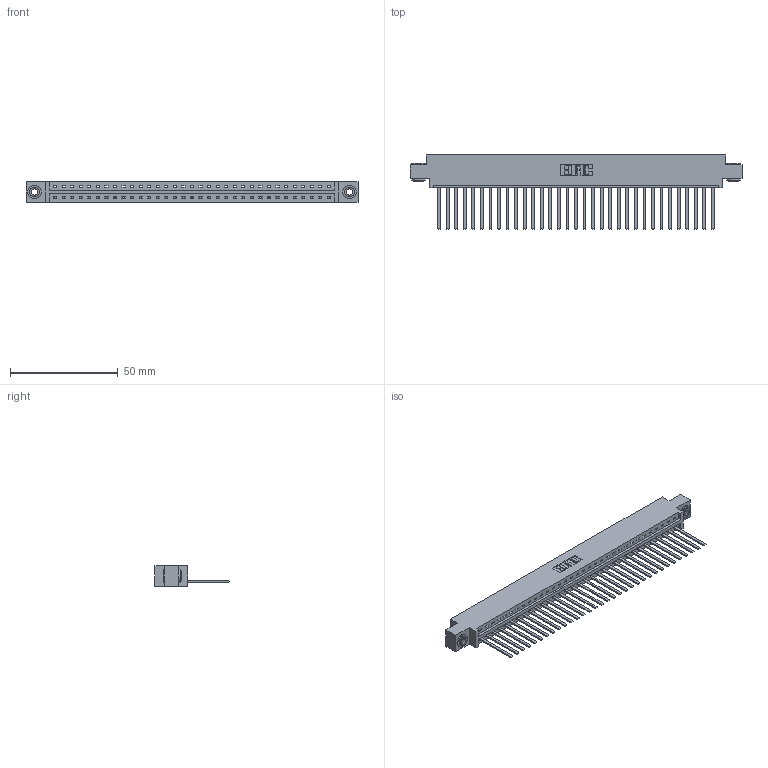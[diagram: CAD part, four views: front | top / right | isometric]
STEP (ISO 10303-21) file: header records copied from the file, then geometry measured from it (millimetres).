
FILE_DESCRIPTION (( 'STEP AP203' ), '1' );
FILE_NAME ('337-033-544-603.STEP', '2019-10-01T11:05:52', ( '' ), ( '' ), 'SwSTEP 2.0', 'SolidWorks 2016', '' );
FILE_SCHEMA (( 'CONFIG_CONTROL_DESIGN' ));
Length unit declared in the file: inch
Products named in the file (4): 345-292-001_345-293-144; 345-250-002_345-250-002-102; 337-033-544-603; 337 Part_0.170 Offset - 0.156 Dia-TH
Assembly tree (36 placements, depth 2):
  337-033-544-603
    337 Part_0.170 Offset - 0.156 Dia-TH
    345-292-001_345-293-144  x33
    345-250-002_345-250-002-102  x2
Bounding box: 153.77 x 34.3 x 9.4 mm (x, y, z)
Volume: 16153.4 mm3; surface area: 18228.6 mm2
Topology: 36 solids, 36 shells, 2004 faces, 6009 edges, 3958 vertices
Faces by surface type: plane 1470, cylinder 526, cone 8
Entity records: 26292 total; most frequent: CARTESIAN_POINT 4556, ORIENTED_EDGE 4518, DIRECTION 3883, EDGE_CURVE 2259, LINE 2111, VECTOR 2111, VERTEX_POINT 1502, AXIS2_PLACEMENT_3D 886
